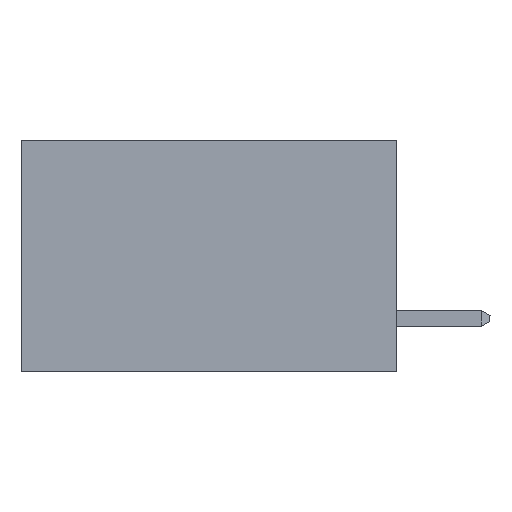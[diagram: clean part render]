
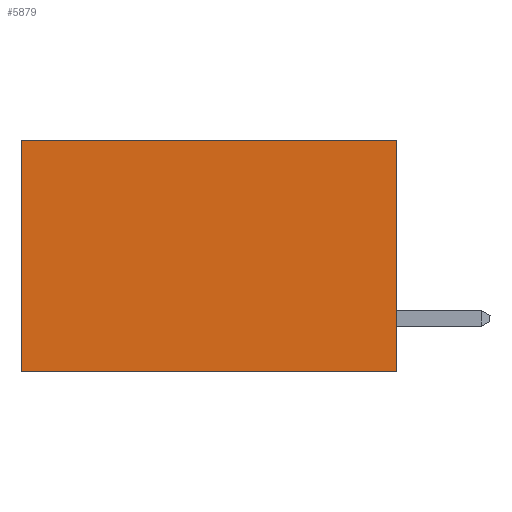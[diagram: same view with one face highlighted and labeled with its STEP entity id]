
A CAD part, left-side view. The second image highlights one B-rep face of the part: STEP entity #5879.
In plain terms, the highlighted planar face has unit normal (-1, 0, 0).
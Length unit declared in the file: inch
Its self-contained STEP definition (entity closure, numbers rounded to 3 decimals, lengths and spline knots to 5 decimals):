
#1147 = DIRECTION ( 'NONE',  ( 0., 0., -1. ) ) ;
#1184 = VECTOR ( 'NONE', #12324, 39.37008 ) ;
#1196 = DIRECTION ( 'NONE',  ( 1., 0., 0. ) ) ;
#1271 = PLANE ( 'NONE',  #13496 ) ;
#1294 = CARTESIAN_POINT ( 'NONE',  ( 0.2615, 0., -0.37 ) ) ;
#1599 = VERTEX_POINT ( 'NONE', #15170 ) ;
#2541 = VERTEX_POINT ( 'NONE', #11193 ) ;
#2814 = VERTEX_POINT ( 'NONE', #12622 ) ;
#3681 = CARTESIAN_POINT ( 'NONE',  ( 0.2615, 0., 0. ) ) ;
#3981 = EDGE_CURVE ( 'NONE', #9253, #2814, #11261, .T. ) ;
#4601 = DIRECTION ( 'NONE',  ( 0., 0., -1. ) ) ;
#4760 = ORIENTED_EDGE ( 'NONE', *, *, #9475, .T. ) ;
#5648 = ORIENTED_EDGE ( 'NONE', *, *, #3981, .F. ) ;
#5879 = ADVANCED_FACE ( 'NONE', ( #16247 ), #1271, .F. ) ;
#6135 = VECTOR ( 'NONE', #8870, 39.37008 ) ;
#6696 = ORIENTED_EDGE ( 'NONE', *, *, #9635, .T. ) ;
#7380 = EDGE_CURVE ( 'NONE', #1599, #9253, #10251, .T. ) ;
#7831 = LINE ( 'NONE', #3681, #10364 ) ;
#8161 = ORIENTED_EDGE ( 'NONE', *, *, #7380, .F. ) ;
#8630 = CARTESIAN_POINT ( 'NONE',  ( 0.2615, 0., -0.37 ) ) ;
#8870 = DIRECTION ( 'NONE',  ( 0., 0., -1. ) ) ;
#9253 = VERTEX_POINT ( 'NONE', #15398 ) ;
#9475 = EDGE_CURVE ( 'NONE', #2541, #2814, #15935, .T. ) ;
#9635 = EDGE_CURVE ( 'NONE', #1599, #2541, #7831, .T. ) ;
#9783 = VECTOR ( 'NONE', #4601, 39.37008 ) ;
#10251 = LINE ( 'NONE', #8630, #6135 ) ;
#10364 = VECTOR ( 'NONE', #13730, 39.37008 ) ;
#10942 = CARTESIAN_POINT ( 'NONE',  ( 0.2615, 0.6, -0.37 ) ) ;
#11193 = CARTESIAN_POINT ( 'NONE',  ( 0.2615, 0.6, 0. ) ) ;
#11261 = LINE ( 'NONE', #12430, #1184 ) ;
#12324 = DIRECTION ( 'NONE',  ( 0., 1., 0. ) ) ;
#12430 = CARTESIAN_POINT ( 'NONE',  ( 0.2615, 0., -0.37 ) ) ;
#12622 = CARTESIAN_POINT ( 'NONE',  ( 0.2615, 0.6, -0.37 ) ) ;
#13496 = AXIS2_PLACEMENT_3D ( 'NONE', #1294, #1196, #1147 ) ;
#13730 = DIRECTION ( 'NONE',  ( 0., 1., 0. ) ) ;
#15156 = EDGE_LOOP ( 'NONE', ( #4760, #5648, #8161, #6696 ) ) ;
#15170 = CARTESIAN_POINT ( 'NONE',  ( 0.2615, 0., 0. ) ) ;
#15398 = CARTESIAN_POINT ( 'NONE',  ( 0.2615, 0., -0.37 ) ) ;
#15935 = LINE ( 'NONE', #10942, #9783 ) ;
#16247 = FACE_OUTER_BOUND ( 'NONE', #15156, .T. ) ;
